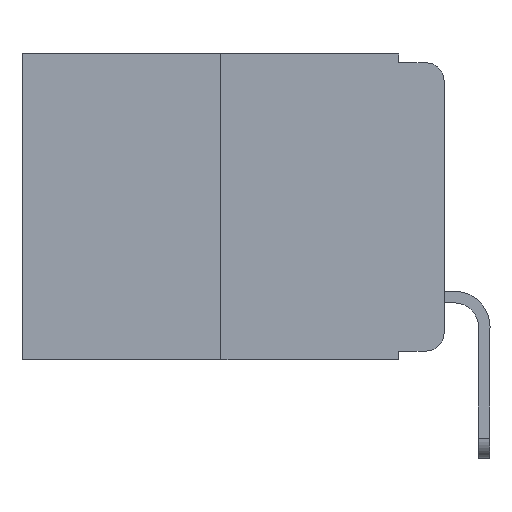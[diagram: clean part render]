
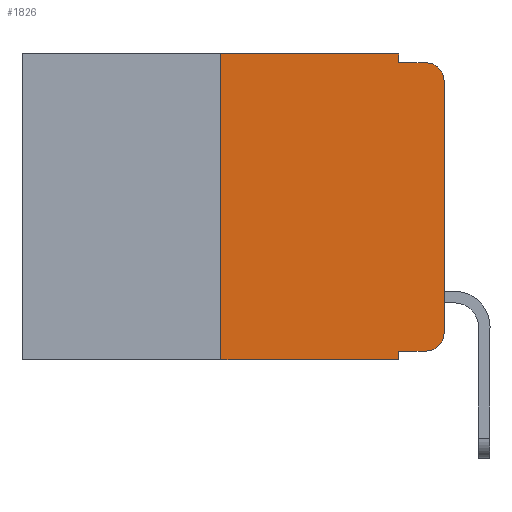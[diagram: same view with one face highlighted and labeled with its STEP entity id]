
A CAD part, left-side view. The second image highlights one B-rep face of the part: STEP entity #1826.
In plain terms, the highlighted planar face has unit normal (-1, 0, 0).
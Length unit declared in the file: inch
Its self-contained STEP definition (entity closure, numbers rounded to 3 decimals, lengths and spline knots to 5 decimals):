
#81 = LINE ( 'NONE', #2181, #5449 ) ;
#315 = CIRCLE ( 'NONE', #11190, 0.02 ) ;
#594 = EDGE_CURVE ( 'NONE', #5050, #3471, #5120, .T. ) ;
#705 = LINE ( 'NONE', #2293, #10717 ) ;
#823 = ORIENTED_EDGE ( 'NONE', *, *, #9169, .T. ) ;
#1099 = VERTEX_POINT ( 'NONE', #13607 ) ;
#1589 = EDGE_LOOP ( 'NONE', ( #11402, #823, #9766, #4640, #12622, #4957, #5283, #10669, #13230, #11565 ) ) ;
#1826 = ADVANCED_FACE ( 'NONE', ( #13489 ), #8804, .F. ) ;
#2107 = EDGE_CURVE ( 'NONE', #5905, #5508, #5548, .T. ) ;
#2181 = CARTESIAN_POINT ( 'NONE',  ( 0., 0.473, -0.343 ) ) ;
#2293 = CARTESIAN_POINT ( 'NONE',  ( 0., 0.051, 0. ) ) ;
#2353 = DIRECTION ( 'NONE',  ( 0., -1., 0. ) ) ;
#2411 = CARTESIAN_POINT ( 'NONE',  ( 0., 0.25, 0. ) ) ;
#2493 = VERTEX_POINT ( 'NONE', #12379 ) ;
#2681 = CARTESIAN_POINT ( 'NONE',  ( 0., 0.02, -0.01 ) ) ;
#2682 = VERTEX_POINT ( 'NONE', #2681 ) ;
#2861 = VERTEX_POINT ( 'NONE', #4306 ) ;
#2874 = DIRECTION ( 'NONE',  ( 0., 0., -1. ) ) ;
#3471 = VERTEX_POINT ( 'NONE', #7602 ) ;
#3507 = DIRECTION ( 'NONE',  ( 0., 0., -1. ) ) ;
#4241 = CARTESIAN_POINT ( 'NONE',  ( 0., 0.473, 0. ) ) ;
#4306 = CARTESIAN_POINT ( 'NONE',  ( 0., 0.051, -0.333 ) ) ;
#4336 = DIRECTION ( 'NONE',  ( 0., 0., 1. ) ) ;
#4381 = CARTESIAN_POINT ( 'NONE',  ( 0., 0.02, -0.333 ) ) ;
#4640 = ORIENTED_EDGE ( 'NONE', *, *, #8848, .F. ) ;
#4706 = DIRECTION ( 'NONE',  ( 1., 0., 0. ) ) ;
#4957 = ORIENTED_EDGE ( 'NONE', *, *, #8021, .F. ) ;
#5009 = LINE ( 'NONE', #10657, #7457 ) ;
#5050 = VERTEX_POINT ( 'NONE', #12162 ) ;
#5056 = DIRECTION ( 'NONE',  ( -1., 0., 0. ) ) ;
#5120 = LINE ( 'NONE', #11337, #13062 ) ;
#5283 = ORIENTED_EDGE ( 'NONE', *, *, #7712, .T. ) ;
#5449 = VECTOR ( 'NONE', #9585, 39.37008 ) ;
#5508 = VERTEX_POINT ( 'NONE', #6871 ) ;
#5548 = CIRCLE ( 'NONE', #12215, 0.02 ) ;
#5583 = DIRECTION ( 'NONE',  ( 0., 0., -1. ) ) ;
#5663 = DIRECTION ( 'NONE',  ( -1., 0., 0. ) ) ;
#5682 = CARTESIAN_POINT ( 'NONE',  ( 0., 0.02, -0.313 ) ) ;
#5905 = VERTEX_POINT ( 'NONE', #4381 ) ;
#6871 = CARTESIAN_POINT ( 'NONE',  ( 0., 0., -0.313 ) ) ;
#7133 = LINE ( 'NONE', #2411, #12047 ) ;
#7419 = VERTEX_POINT ( 'NONE', #11175 ) ;
#7457 = VECTOR ( 'NONE', #3507, 39.37008 ) ;
#7602 = CARTESIAN_POINT ( 'NONE',  ( 0., 0.051, 0. ) ) ;
#7707 = CARTESIAN_POINT ( 'NONE',  ( 0., 0.051, -0.01 ) ) ;
#7712 = EDGE_CURVE ( 'NONE', #2493, #10654, #81, .T. ) ;
#7838 = EDGE_CURVE ( 'NONE', #2861, #5905, #9342, .T. ) ;
#7937 = EDGE_CURVE ( 'NONE', #2861, #10654, #5009, .T. ) ;
#8021 = EDGE_CURVE ( 'NONE', #2493, #5050, #7133, .T. ) ;
#8599 = DIRECTION ( 'NONE',  ( 0., -1., 0. ) ) ;
#8804 = PLANE ( 'NONE',  #8805 ) ;
#8805 = AXIS2_PLACEMENT_3D ( 'NONE', #4241, #4706, #2874 ) ;
#8848 = EDGE_CURVE ( 'NONE', #3471, #7419, #705, .T. ) ;
#8864 = LINE ( 'NONE', #10427, #11143 ) ;
#8865 = EDGE_CURVE ( 'NONE', #7419, #2682, #13604, .T. ) ;
#9169 = EDGE_CURVE ( 'NONE', #1099, #2682, #315, .T. ) ;
#9342 = LINE ( 'NONE', #9554, #10715 ) ;
#9436 = EDGE_CURVE ( 'NONE', #5508, #1099, #8864, .T. ) ;
#9554 = CARTESIAN_POINT ( 'NONE',  ( 0., 0.051, -0.333 ) ) ;
#9585 = DIRECTION ( 'NONE',  ( 0., -1., 0. ) ) ;
#9766 = ORIENTED_EDGE ( 'NONE', *, *, #8865, .F. ) ;
#9773 = DIRECTION ( 'NONE',  ( 0., 0., 1. ) ) ;
#10427 = CARTESIAN_POINT ( 'NONE',  ( 0., 0., 0. ) ) ;
#10654 = VERTEX_POINT ( 'NONE', #12831 ) ;
#10657 = CARTESIAN_POINT ( 'NONE',  ( 0., 0.051, 0. ) ) ;
#10666 = DIRECTION ( 'NONE',  ( 0., -1., 0. ) ) ;
#10669 = ORIENTED_EDGE ( 'NONE', *, *, #7937, .F. ) ;
#10715 = VECTOR ( 'NONE', #8599, 39.37008 ) ;
#10717 = VECTOR ( 'NONE', #11613, 39.37008 ) ;
#11089 = CARTESIAN_POINT ( 'NONE',  ( 0., 0.02, -0.03 ) ) ;
#11143 = VECTOR ( 'NONE', #4336, 39.37008 ) ;
#11175 = CARTESIAN_POINT ( 'NONE',  ( 0., 0.051, -0.01 ) ) ;
#11190 = AXIS2_PLACEMENT_3D ( 'NONE', #11089, #5056, #12049 ) ;
#11337 = CARTESIAN_POINT ( 'NONE',  ( 0., 0.473, 0. ) ) ;
#11402 = ORIENTED_EDGE ( 'NONE', *, *, #9436, .T. ) ;
#11565 = ORIENTED_EDGE ( 'NONE', *, *, #2107, .T. ) ;
#11613 = DIRECTION ( 'NONE',  ( 0., 0., -1. ) ) ;
#12047 = VECTOR ( 'NONE', #9773, 39.37008 ) ;
#12049 = DIRECTION ( 'NONE',  ( 0., 0., -1. ) ) ;
#12162 = CARTESIAN_POINT ( 'NONE',  ( 0., 0.25, 0. ) ) ;
#12215 = AXIS2_PLACEMENT_3D ( 'NONE', #5682, #5663, #5583 ) ;
#12379 = CARTESIAN_POINT ( 'NONE',  ( 0., 0.25, -0.343 ) ) ;
#12622 = ORIENTED_EDGE ( 'NONE', *, *, #594, .F. ) ;
#12831 = CARTESIAN_POINT ( 'NONE',  ( 0., 0.051, -0.343 ) ) ;
#12972 = VECTOR ( 'NONE', #2353, 39.37008 ) ;
#13062 = VECTOR ( 'NONE', #10666, 39.37008 ) ;
#13230 = ORIENTED_EDGE ( 'NONE', *, *, #7838, .T. ) ;
#13489 = FACE_OUTER_BOUND ( 'NONE', #1589, .T. ) ;
#13604 = LINE ( 'NONE', #7707, #12972 ) ;
#13607 = CARTESIAN_POINT ( 'NONE',  ( 0., 0., -0.03 ) ) ;
